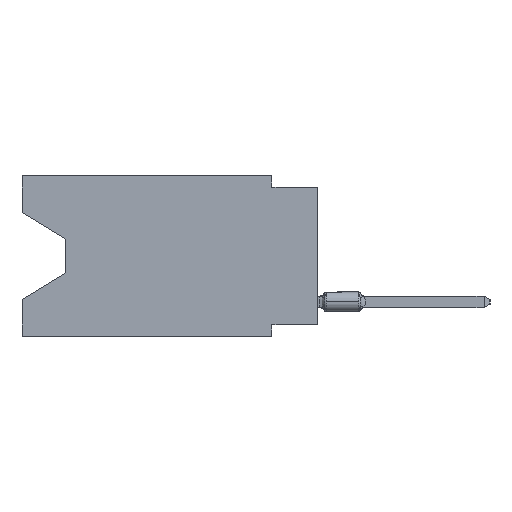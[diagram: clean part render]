
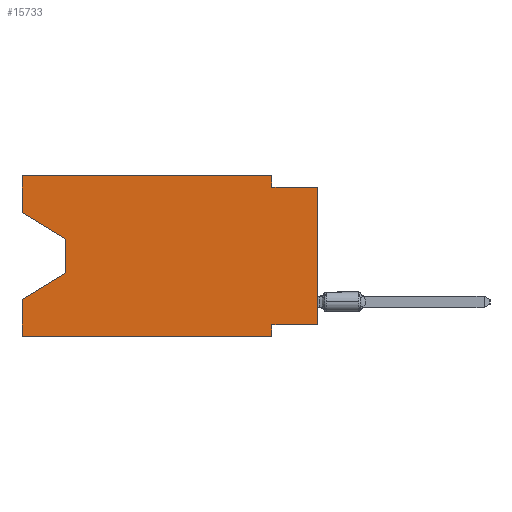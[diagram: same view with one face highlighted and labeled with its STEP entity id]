
A CAD part, left-side view. The second image highlights one B-rep face of the part: STEP entity #15733.
In plain terms, the highlighted planar face has unit normal (-1, 0, 0).
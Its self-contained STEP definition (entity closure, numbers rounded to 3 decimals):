
#178 = PLANE ( 'NONE',  #7429 ) ;
#448 = DIRECTION ( 'NONE',  ( 0., 0., 1. ) ) ;
#505 = DIRECTION ( 'NONE',  ( 0., -1., 0. ) ) ;
#510 = ORIENTED_EDGE ( 'NONE', *, *, #11559, .T. ) ;
#589 = LINE ( 'NONE', #18599, #15801 ) ;
#986 = CARTESIAN_POINT ( 'NONE',  ( 0., 16.383, -2.038 ) ) ;
#1121 = VECTOR ( 'NONE', #14109, 1000. ) ;
#1150 = VERTEX_POINT ( 'NONE', #27707 ) ;
#1183 = LINE ( 'NONE', #3233, #23490 ) ;
#1237 = ORIENTED_EDGE ( 'NONE', *, *, #13010, .F. ) ;
#1340 = CARTESIAN_POINT ( 'NONE',  ( 0., 2.54, -8.255 ) ) ;
#1923 = CARTESIAN_POINT ( 'NONE',  ( 0., 2.54, -0.635 ) ) ;
#2013 = CARTESIAN_POINT ( 'NONE',  ( 0., 13.97, -3.505 ) ) ;
#2612 = VERTEX_POINT ( 'NONE', #2013 ) ;
#3144 = VERTEX_POINT ( 'NONE', #18182 ) ;
#3233 = CARTESIAN_POINT ( 'NONE',  ( 0., 0., 0. ) ) ;
#3585 = CARTESIAN_POINT ( 'NONE',  ( 0., 2.54, 0. ) ) ;
#3859 = ORIENTED_EDGE ( 'NONE', *, *, #12253, .F. ) ;
#3991 = VECTOR ( 'NONE', #11648, 1000. ) ;
#4209 = VECTOR ( 'NONE', #505, 1000. ) ;
#4512 = LINE ( 'NONE', #22531, #6325 ) ;
#4594 = CARTESIAN_POINT ( 'NONE',  ( 0., 0., -0.635 ) ) ;
#5197 = EDGE_CURVE ( 'NONE', #27126, #8895, #27954, .T. ) ;
#5859 = CARTESIAN_POINT ( 'NONE',  ( 0., 16.383, 0. ) ) ;
#6236 = CARTESIAN_POINT ( 'NONE',  ( 0., 2.54, -8.89 ) ) ;
#6325 = VECTOR ( 'NONE', #15793, 1000. ) ;
#6429 = EDGE_CURVE ( 'NONE', #27126, #11198, #1183, .T. ) ;
#6814 = LINE ( 'NONE', #13556, #3991 ) ;
#7371 = CARTESIAN_POINT ( 'NONE',  ( 0., 2.54, -8.89 ) ) ;
#7429 = AXIS2_PLACEMENT_3D ( 'NONE', #9109, #26971, #18183 ) ;
#7518 = LINE ( 'NONE', #7371, #1121 ) ;
#7759 = LINE ( 'NONE', #5859, #28275 ) ;
#7900 = VERTEX_POINT ( 'NONE', #16480 ) ;
#8317 = EDGE_CURVE ( 'NONE', #8895, #12716, #7518, .T. ) ;
#8895 = VERTEX_POINT ( 'NONE', #1340 ) ;
#9109 = CARTESIAN_POINT ( 'NONE',  ( 0., 16.383, 0. ) ) ;
#9927 = ORIENTED_EDGE ( 'NONE', *, *, #25515, .T. ) ;
#10150 = ORIENTED_EDGE ( 'NONE', *, *, #13974, .F. ) ;
#10395 = DIRECTION ( 'NONE',  ( 0., -1., 0. ) ) ;
#11198 = VERTEX_POINT ( 'NONE', #23065 ) ;
#11205 = ORIENTED_EDGE ( 'NONE', *, *, #18455, .F. ) ;
#11559 = EDGE_CURVE ( 'NONE', #12846, #7900, #23175, .T. ) ;
#11648 = DIRECTION ( 'NONE',  ( 0., 0., 1. ) ) ;
#12004 = CARTESIAN_POINT ( 'NONE',  ( 0., 2.54, 0. ) ) ;
#12253 = EDGE_CURVE ( 'NONE', #3144, #21649, #6814, .T. ) ;
#12287 = CARTESIAN_POINT ( 'NONE',  ( 0., 0., -8.255 ) ) ;
#12716 = VERTEX_POINT ( 'NONE', #6236 ) ;
#12846 = VERTEX_POINT ( 'NONE', #27017 ) ;
#13010 = EDGE_CURVE ( 'NONE', #1150, #7900, #589, .T. ) ;
#13556 = CARTESIAN_POINT ( 'NONE',  ( 0., 16.383, 0. ) ) ;
#13974 = EDGE_CURVE ( 'NONE', #24098, #18108, #21601, .T. ) ;
#14109 = DIRECTION ( 'NONE',  ( 0., 0., -1. ) ) ;
#15378 = VECTOR ( 'NONE', #19261, 1000. ) ;
#15733 = ADVANCED_FACE ( 'NONE', ( #20238 ), #178, .F. ) ;
#15793 = DIRECTION ( 'NONE',  ( 0., -1., 0. ) ) ;
#15801 = VECTOR ( 'NONE', #448, 1000. ) ;
#16088 = DIRECTION ( 'NONE',  ( 0., 0., -1. ) ) ;
#16290 = CARTESIAN_POINT ( 'NONE',  ( 0., 13.97, -5.385 ) ) ;
#16480 = CARTESIAN_POINT ( 'NONE',  ( 0., 16.383, -6.852 ) ) ;
#16606 = EDGE_CURVE ( 'NONE', #18108, #11198, #20575, .T. ) ;
#16621 = ORIENTED_EDGE ( 'NONE', *, *, #6429, .T. ) ;
#16649 = DIRECTION ( 'NONE',  ( 0., -0.855, -0.519 ) ) ;
#16897 = ORIENTED_EDGE ( 'NONE', *, *, #16606, .F. ) ;
#17977 = LINE ( 'NONE', #18563, #20368 ) ;
#18050 = VECTOR ( 'NONE', #16649, 1000. ) ;
#18108 = VERTEX_POINT ( 'NONE', #1923 ) ;
#18182 = CARTESIAN_POINT ( 'NONE',  ( 0., 16.383, -2.038 ) ) ;
#18183 = DIRECTION ( 'NONE',  ( 0., 0., -1. ) ) ;
#18455 = EDGE_CURVE ( 'NONE', #21649, #24098, #7759, .T. ) ;
#18563 = CARTESIAN_POINT ( 'NONE',  ( 0., 13.97, -3.505 ) ) ;
#18599 = CARTESIAN_POINT ( 'NONE',  ( 0., 16.383, 0. ) ) ;
#18832 = ORIENTED_EDGE ( 'NONE', *, *, #8317, .F. ) ;
#19035 = DIRECTION ( 'NONE',  ( 0., 1., 0. ) ) ;
#19136 = ORIENTED_EDGE ( 'NONE', *, *, #19850, .T. ) ;
#19261 = DIRECTION ( 'NONE',  ( 0., 0., -1. ) ) ;
#19850 = EDGE_CURVE ( 'NONE', #3144, #2612, #21349, .T. ) ;
#20238 = FACE_OUTER_BOUND ( 'NONE', #26693, .T. ) ;
#20368 = VECTOR ( 'NONE', #16088, 1000. ) ;
#20575 = LINE ( 'NONE', #4594, #4209 ) ;
#21349 = LINE ( 'NONE', #986, #18050 ) ;
#21601 = LINE ( 'NONE', #3585, #15378 ) ;
#21649 = VERTEX_POINT ( 'NONE', #23808 ) ;
#22220 = ORIENTED_EDGE ( 'NONE', *, *, #5197, .F. ) ;
#22531 = CARTESIAN_POINT ( 'NONE',  ( 0., 16.383, -8.89 ) ) ;
#23065 = CARTESIAN_POINT ( 'NONE',  ( 0., 0., -0.635 ) ) ;
#23175 = LINE ( 'NONE', #16290, #26878 ) ;
#23490 = VECTOR ( 'NONE', #25494, 1000. ) ;
#23808 = CARTESIAN_POINT ( 'NONE',  ( 0., 16.383, 0. ) ) ;
#24098 = VERTEX_POINT ( 'NONE', #12004 ) ;
#24161 = ORIENTED_EDGE ( 'NONE', *, *, #25593, .T. ) ;
#24348 = CARTESIAN_POINT ( 'NONE',  ( 0., 0., -8.255 ) ) ;
#25494 = DIRECTION ( 'NONE',  ( 0., 0., 1. ) ) ;
#25515 = EDGE_CURVE ( 'NONE', #1150, #12716, #4512, .T. ) ;
#25593 = EDGE_CURVE ( 'NONE', #2612, #12846, #17977, .T. ) ;
#25795 = VECTOR ( 'NONE', #19035, 1000. ) ;
#26693 = EDGE_LOOP ( 'NONE', ( #19136, #24161, #510, #1237, #9927, #18832, #22220, #16621, #16897, #10150, #11205, #3859 ) ) ;
#26878 = VECTOR ( 'NONE', #27262, 1000. ) ;
#26971 = DIRECTION ( 'NONE',  ( 1., 0., 0. ) ) ;
#27017 = CARTESIAN_POINT ( 'NONE',  ( 0., 13.97, -5.385 ) ) ;
#27126 = VERTEX_POINT ( 'NONE', #24348 ) ;
#27262 = DIRECTION ( 'NONE',  ( 0., 0.855, -0.519 ) ) ;
#27707 = CARTESIAN_POINT ( 'NONE',  ( 0., 16.383, -8.89 ) ) ;
#27954 = LINE ( 'NONE', #12287, #25795 ) ;
#28275 = VECTOR ( 'NONE', #10395, 1000. ) ;
